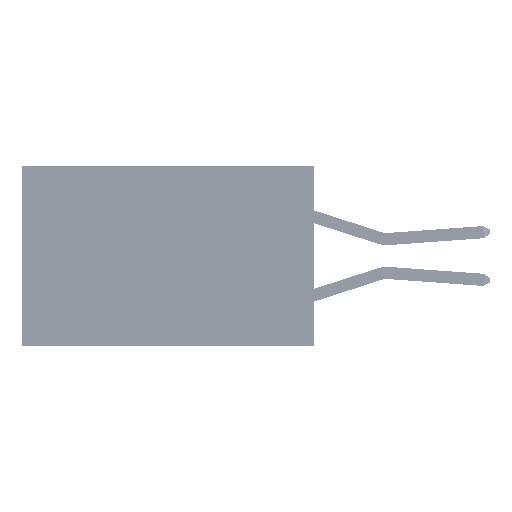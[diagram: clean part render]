
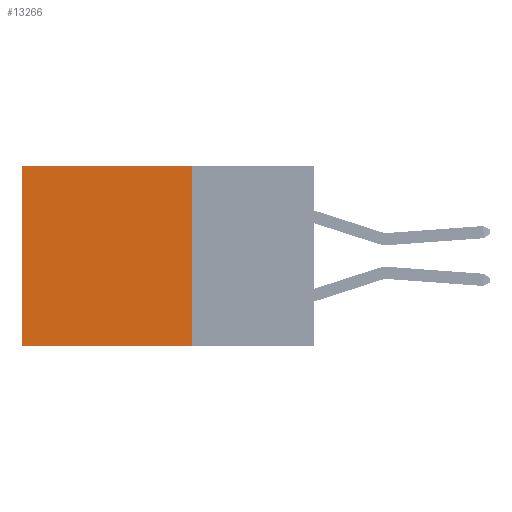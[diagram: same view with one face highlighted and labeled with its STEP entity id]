
A CAD part, left-side view. The second image highlights one B-rep face of the part: STEP entity #13266.
In plain terms, the highlighted planar face has unit normal (-1, 0, 0).
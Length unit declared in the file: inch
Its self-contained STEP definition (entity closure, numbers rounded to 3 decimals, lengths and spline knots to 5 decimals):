
#1781 = CARTESIAN_POINT ( 'NONE',  ( 0.2875, 0.25, 0. ) ) ;
#3197 = ORIENTED_EDGE ( 'NONE', *, *, #32410, .T. ) ;
#9963 = VERTEX_POINT ( 'NONE', #43968 ) ;
#10058 = CARTESIAN_POINT ( 'NONE',  ( 0.2875, 0.25, 0. ) ) ;
#10069 = DIRECTION ( 'NONE',  ( 0., 0., -1. ) ) ;
#10511 = CARTESIAN_POINT ( 'NONE',  ( 0.2875, 0.6, -0.37 ) ) ;
#11800 = DIRECTION ( 'NONE',  ( 0., 0., -1. ) ) ;
#12478 = FACE_OUTER_BOUND ( 'NONE', #22759, .T. ) ;
#13266 = ADVANCED_FACE ( 'NONE', ( #12478 ), #21915, .F. ) ;
#13342 = VECTOR ( 'NONE', #10069, 39.37008 ) ;
#14458 = CARTESIAN_POINT ( 'NONE',  ( 0.2875, 0.25, -0.37 ) ) ;
#16298 = CARTESIAN_POINT ( 'NONE',  ( 0.2875, 0.6, 0. ) ) ;
#16831 = LINE ( 'NONE', #1781, #33295 ) ;
#20264 = VERTEX_POINT ( 'NONE', #10511 ) ;
#20389 = AXIS2_PLACEMENT_3D ( 'NONE', #10058, #30009, #50439 ) ;
#21436 = ORIENTED_EDGE ( 'NONE', *, *, #52200, .F. ) ;
#21915 = PLANE ( 'NONE',  #20389 ) ;
#22583 = ORIENTED_EDGE ( 'NONE', *, *, #46773, .F. ) ;
#22759 = EDGE_LOOP ( 'NONE', ( #37477, #21436, #22583, #3197 ) ) ;
#23462 = LINE ( 'NONE', #50446, #13342 ) ;
#25970 = VECTOR ( 'NONE', #37995, 39.37008 ) ;
#28016 = VECTOR ( 'NONE', #11800, 39.37008 ) ;
#28540 = CARTESIAN_POINT ( 'NONE',  ( 0.2875, 0.25, 0. ) ) ;
#30009 = DIRECTION ( 'NONE',  ( 1., 0., 0. ) ) ;
#32410 = EDGE_CURVE ( 'NONE', #9963, #35455, #16831, .T. ) ;
#33295 = VECTOR ( 'NONE', #46806, 39.37008 ) ;
#35455 = VERTEX_POINT ( 'NONE', #16298 ) ;
#35640 = LINE ( 'NONE', #28540, #28016 ) ;
#36718 = LINE ( 'NONE', #50969, #25970 ) ;
#37477 = ORIENTED_EDGE ( 'NONE', *, *, #52225, .T. ) ;
#37995 = DIRECTION ( 'NONE',  ( 0., 1., 0. ) ) ;
#43968 = CARTESIAN_POINT ( 'NONE',  ( 0.2875, 0.25, 0. ) ) ;
#45909 = VERTEX_POINT ( 'NONE', #14458 ) ;
#46773 = EDGE_CURVE ( 'NONE', #9963, #45909, #35640, .T. ) ;
#46806 = DIRECTION ( 'NONE',  ( 0., 1., 0. ) ) ;
#50439 = DIRECTION ( 'NONE',  ( 0., 0., -1. ) ) ;
#50446 = CARTESIAN_POINT ( 'NONE',  ( 0.2875, 0.6, 0. ) ) ;
#50969 = CARTESIAN_POINT ( 'NONE',  ( 0.2875, 0.25, -0.37 ) ) ;
#52200 = EDGE_CURVE ( 'NONE', #45909, #20264, #36718, .T. ) ;
#52225 = EDGE_CURVE ( 'NONE', #35455, #20264, #23462, .T. ) ;
